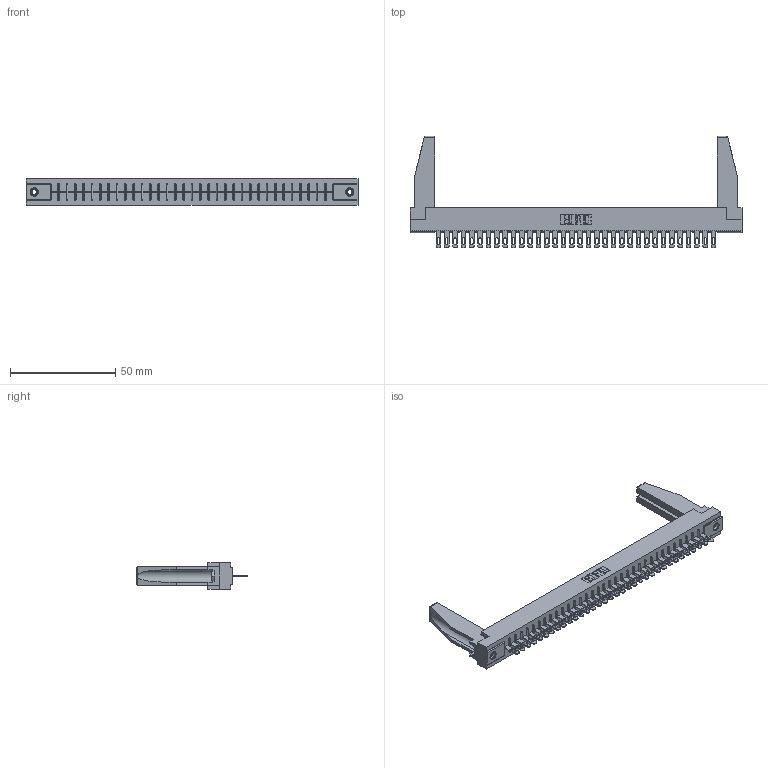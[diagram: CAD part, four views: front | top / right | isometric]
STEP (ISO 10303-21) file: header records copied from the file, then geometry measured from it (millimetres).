
FILE_DESCRIPTION (( 'STEP AP203' ), '1' );
FILE_NAME ('306-034-400-178.STEP', '2020-09-22T03:15:01', ( '' ), ( '' ), 'SwSTEP 2.0', 'SolidWorks 2020', '' );
FILE_SCHEMA (( 'CONFIG_CONTROL_DESIGN' ));
Length unit declared in the file: inch
Products named in the file (5): 345-250-001_345-250-001-102; 306 Part_.156 Dia; 306-034-400-178; 306-290-001_100; 307-220-078
Assembly tree (39 placements, depth 2):
  306-034-400-178
    306 Part_.156 Dia
    306-290-001_100  x34
    345-250-001_345-250-001-102  x2
    307-220-078  x2
Bounding box: 157.73 x 52.91 x 12.7 mm (x, y, z)
Volume: 21471.5 mm3; surface area: 22286.2 mm2
Topology: 39 solids, 39 shells, 2830 faces, 7956 edges, 5112 vertices
Faces by surface type: plane 1852, cylinder 826, sphere 136, cone 12, torus 4
Entity records: 35346 total; most frequent: CARTESIAN_POINT 5935, ORIENTED_EDGE 5842, DIRECTION 5805, EDGE_CURVE 2921, VECTOR 2281, LINE 2281, VERTEX_POINT 1850, AXIS2_PLACEMENT_3D 1762
